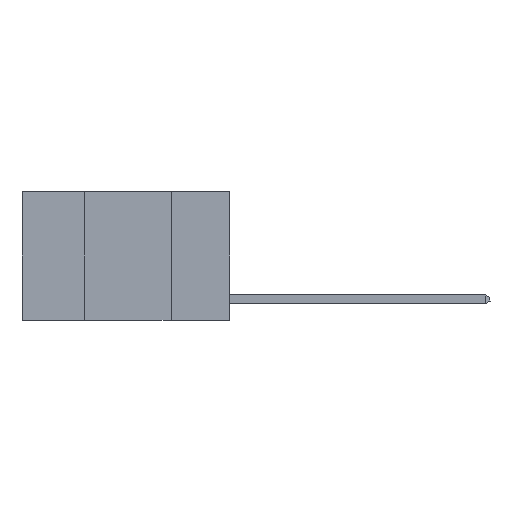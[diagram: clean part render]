
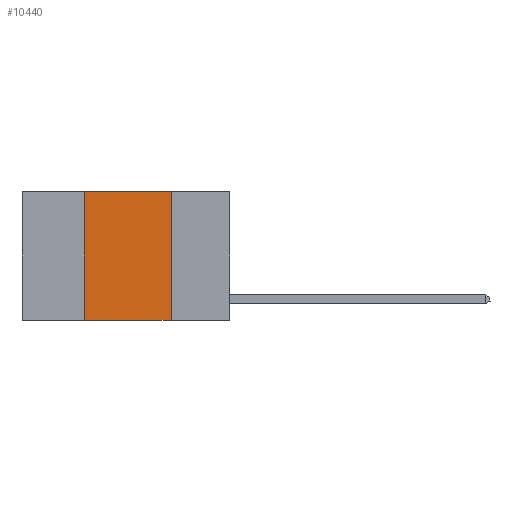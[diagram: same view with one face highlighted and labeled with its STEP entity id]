
A CAD part, left-side view. The second image highlights one B-rep face of the part: STEP entity #10440.
In plain terms, the highlighted planar face has unit normal (-1, 0, 0).
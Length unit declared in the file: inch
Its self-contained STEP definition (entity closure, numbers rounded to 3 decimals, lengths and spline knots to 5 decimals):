
#180 = VERTEX_POINT ( 'NONE', #14811 ) ;
#184 = CARTESIAN_POINT ( 'NONE',  ( 0., 0.17, -0.37 ) ) ;
#392 = LINE ( 'NONE', #12256, #6015 ) ;
#875 = CARTESIAN_POINT ( 'NONE',  ( 0., 0.6, 0. ) ) ;
#1080 = EDGE_LOOP ( 'NONE', ( #7422, #4203, #14466, #4500 ) ) ;
#1082 = CARTESIAN_POINT ( 'NONE',  ( 0., 0.42, 0. ) ) ;
#1315 = LINE ( 'NONE', #5765, #12827 ) ;
#1443 = EDGE_CURVE ( 'NONE', #4243, #180, #2012, .T. ) ;
#2012 = LINE ( 'NONE', #6268, #9923 ) ;
#3104 = EDGE_CURVE ( 'NONE', #17063, #12025, #1315, .T. ) ;
#3182 = AXIS2_PLACEMENT_3D ( 'NONE', #875, #15648, #4046 ) ;
#3514 = CARTESIAN_POINT ( 'NONE',  ( 0., 0.42, 0. ) ) ;
#3842 = DIRECTION ( 'NONE',  ( 0., 0., 1. ) ) ;
#4046 = DIRECTION ( 'NONE',  ( 0., 0., -1. ) ) ;
#4203 = ORIENTED_EDGE ( 'NONE', *, *, #1443, .F. ) ;
#4243 = VERTEX_POINT ( 'NONE', #3514 ) ;
#4500 = ORIENTED_EDGE ( 'NONE', *, *, #3104, .T. ) ;
#5765 = CARTESIAN_POINT ( 'NONE',  ( 0., 0.6, -0.37 ) ) ;
#6015 = VECTOR ( 'NONE', #9256, 39.37008 ) ;
#6268 = CARTESIAN_POINT ( 'NONE',  ( 0., 0.6, 0. ) ) ;
#6725 = VECTOR ( 'NONE', #3842, 39.37008 ) ;
#7422 = ORIENTED_EDGE ( 'NONE', *, *, #11532, .F. ) ;
#8372 = LINE ( 'NONE', #1082, #6725 ) ;
#9256 = DIRECTION ( 'NONE',  ( 0., 0., -1. ) ) ;
#9923 = VECTOR ( 'NONE', #15222, 39.37008 ) ;
#10192 = CARTESIAN_POINT ( 'NONE',  ( 0., 0.42, -0.37 ) ) ;
#10440 = ADVANCED_FACE ( 'NONE', ( #14399 ), #11184, .F. ) ;
#11184 = PLANE ( 'NONE',  #3182 ) ;
#11532 = EDGE_CURVE ( 'NONE', #180, #12025, #392, .T. ) ;
#11810 = DIRECTION ( 'NONE',  ( 0., -1., 0. ) ) ;
#12025 = VERTEX_POINT ( 'NONE', #184 ) ;
#12256 = CARTESIAN_POINT ( 'NONE',  ( 0., 0.17, 0. ) ) ;
#12827 = VECTOR ( 'NONE', #11810, 39.37008 ) ;
#13540 = EDGE_CURVE ( 'NONE', #17063, #4243, #8372, .T. ) ;
#14399 = FACE_OUTER_BOUND ( 'NONE', #1080, .T. ) ;
#14466 = ORIENTED_EDGE ( 'NONE', *, *, #13540, .F. ) ;
#14811 = CARTESIAN_POINT ( 'NONE',  ( 0., 0.17, 0. ) ) ;
#15222 = DIRECTION ( 'NONE',  ( 0., -1., 0. ) ) ;
#15648 = DIRECTION ( 'NONE',  ( 1., 0., 0. ) ) ;
#17063 = VERTEX_POINT ( 'NONE', #10192 ) ;
